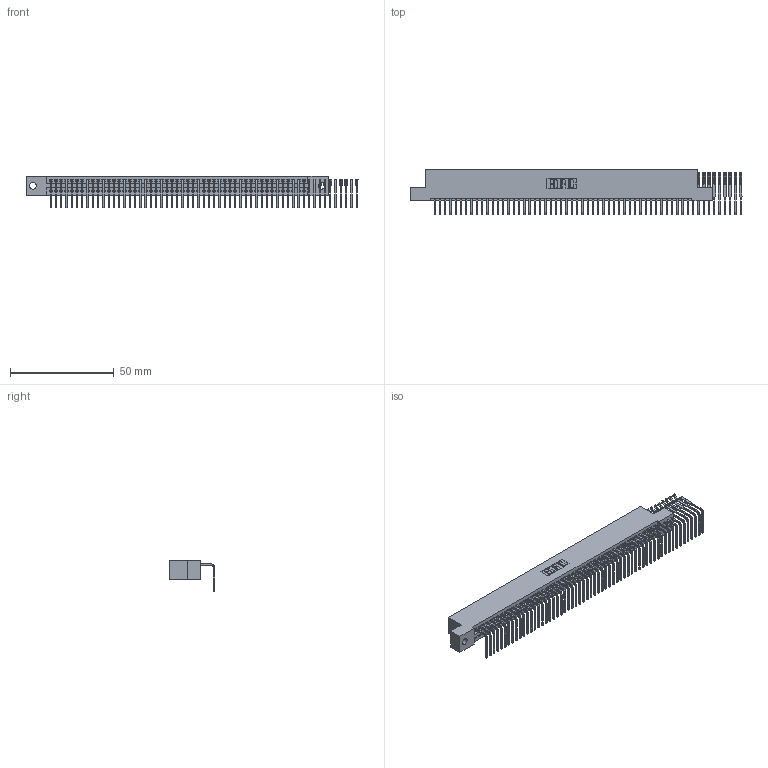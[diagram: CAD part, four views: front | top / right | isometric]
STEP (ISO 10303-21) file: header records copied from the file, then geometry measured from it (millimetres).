
FILE_DESCRIPTION (( 'STEP AP203' ), '1' );
FILE_NAME ('345-059-558-102.STEP', '2019-10-10T20:18:24', ( '' ), ( '' ), 'SwSTEP 2.0', 'SolidWorks 2016', '' );
FILE_SCHEMA (( 'CONFIG_CONTROL_DESIGN' ));
Length unit declared in the file: inch
Products named in the file (3): 345 Part_Flush Mounting Lugs - 0.128 Dia; 345-292-001_558 Tail - 2; 345-059-558-102
Assembly tree (60 placements, depth 2):
  345-059-558-102
    345 Part_Flush Mounting Lugs - 0.128 Dia
    345-292-001_558 Tail - 2  x59
Bounding box: 159.83 x 21.83 x 15.37 mm (x, y, z)
Volume: 14167.5 mm3; surface area: 20414.2 mm2
Topology: 60 solids, 60 shells, 3506 faces, 10539 edges, 6946 vertices
Faces by surface type: plane 2418, cylinder 1088
Entity records: 36343 total; most frequent: CARTESIAN_POINT 6257, ORIENTED_EDGE 6230, DIRECTION 5465, EDGE_CURVE 3115, LINE 2787, VECTOR 2787, VERTEX_POINT 2074, AXIS2_PLACEMENT_3D 1339
